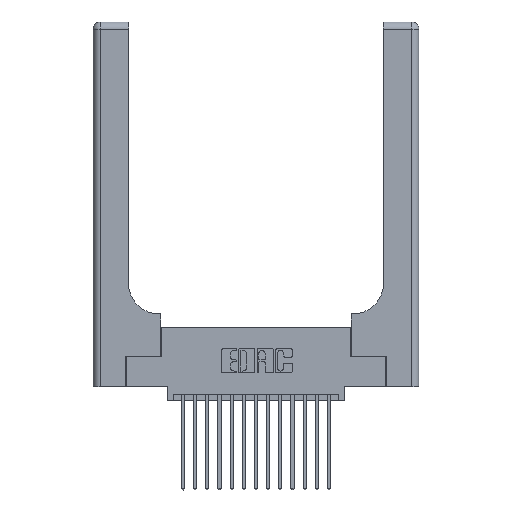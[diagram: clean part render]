
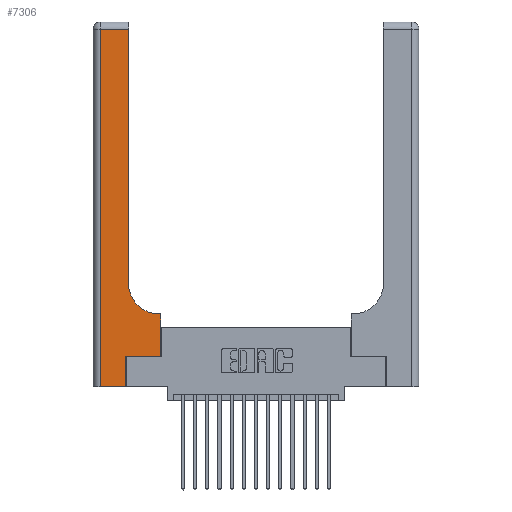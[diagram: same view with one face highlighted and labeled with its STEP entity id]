
A CAD part, top view. The second image highlights one B-rep face of the part: STEP entity #7306.
In plain terms, the highlighted planar face has unit normal (0, 0, 1).
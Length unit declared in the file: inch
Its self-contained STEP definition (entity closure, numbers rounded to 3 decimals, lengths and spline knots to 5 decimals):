
#80 = ORIENTED_EDGE ( 'NONE', *, *, #18007, .T. ) ;
#133 = CARTESIAN_POINT ( 'NONE',  ( 0.2915, 0.85, 0.37 ) ) ;
#310 = CARTESIAN_POINT ( 'NONE',  ( 0.5415, 0.6, 0.37 ) ) ;
#951 = VECTOR ( 'NONE', #5493, 39.37008 ) ;
#1789 = CARTESIAN_POINT ( 'NONE',  ( 0.269, 0., 0.37 ) ) ;
#2284 = LINE ( 'NONE', #10333, #10471 ) ;
#2875 = VECTOR ( 'NONE', #17183, 39.37008 ) ;
#3182 = VERTEX_POINT ( 'NONE', #1789 ) ;
#3317 = EDGE_CURVE ( 'NONE', #3914, #3883, #15483, .T. ) ;
#3883 = VERTEX_POINT ( 'NONE', #9594 ) ;
#3914 = VERTEX_POINT ( 'NONE', #18693 ) ;
#3948 = CARTESIAN_POINT ( 'NONE',  ( 0.5585, 0.25, 0.37 ) ) ;
#4792 = AXIS2_PLACEMENT_3D ( 'NONE', #16618, #9261, #6582 ) ;
#5071 = CARTESIAN_POINT ( 'NONE',  ( 0.2915, 2.94, 0.37 ) ) ;
#5115 = VERTEX_POINT ( 'NONE', #3948 ) ;
#5223 = FACE_OUTER_BOUND ( 'NONE', #6684, .T. ) ;
#5493 = DIRECTION ( 'NONE',  ( 0., 1., 0. ) ) ;
#5684 = ORIENTED_EDGE ( 'NONE', *, *, #13061, .T. ) ;
#6031 = DIRECTION ( 'NONE',  ( 0., 1., 0. ) ) ;
#6466 = CARTESIAN_POINT ( 'NONE',  ( 0.5585, 0.6, 0.37 ) ) ;
#6493 = CARTESIAN_POINT ( 'NONE',  ( 0., 0., 0.37 ) ) ;
#6582 = DIRECTION ( 'NONE',  ( 1., 0., 0. ) ) ;
#6594 = CARTESIAN_POINT ( 'NONE',  ( 0.269, 0.25, 0.37 ) ) ;
#6619 = CARTESIAN_POINT ( 'NONE',  ( 0., 3., 0.37 ) ) ;
#6684 = EDGE_LOOP ( 'NONE', ( #7973, #14461, #9759, #18737, #5684, #13299, #80, #12429, #9542 ) ) ;
#6760 = DIRECTION ( 'NONE',  ( 1., 0., 0. ) ) ;
#7249 = DIRECTION ( 'NONE',  ( -1., 0., 0. ) ) ;
#7306 = ADVANCED_FACE ( 'NONE', ( #5223 ), #15540, .F. ) ;
#7374 = EDGE_CURVE ( 'NONE', #9875, #18195, #12712, .T. ) ;
#7973 = ORIENTED_EDGE ( 'NONE', *, *, #11420, .T. ) ;
#8090 = DIRECTION ( 'NONE',  ( 1., 0., 0. ) ) ;
#8292 = CARTESIAN_POINT ( 'NONE',  ( 0.06, 3., 0.37 ) ) ;
#8516 = AXIS2_PLACEMENT_3D ( 'NONE', #6619, #12692, #11057 ) ;
#8570 = DIRECTION ( 'NONE',  ( -1., 0., 0. ) ) ;
#9261 = DIRECTION ( 'NONE',  ( 0., 0., -1. ) ) ;
#9511 = VECTOR ( 'NONE', #8570, 39.37008 ) ;
#9542 = ORIENTED_EDGE ( 'NONE', *, *, #7374, .T. ) ;
#9594 = CARTESIAN_POINT ( 'NONE',  ( 0.06, 0., 0.37 ) ) ;
#9759 = ORIENTED_EDGE ( 'NONE', *, *, #3317, .T. ) ;
#9875 = VERTEX_POINT ( 'NONE', #310 ) ;
#10333 = CARTESIAN_POINT ( 'NONE',  ( 0., 2.94, 0.37 ) ) ;
#10471 = VECTOR ( 'NONE', #7249, 39.37008 ) ;
#10490 = VECTOR ( 'NONE', #6760, 39.37008 ) ;
#10528 = VERTEX_POINT ( 'NONE', #6466 ) ;
#10738 = VERTEX_POINT ( 'NONE', #14190 ) ;
#10763 = VECTOR ( 'NONE', #17199, 39.37008 ) ;
#11023 = CARTESIAN_POINT ( 'NONE',  ( 0.5585, 0.25, 0.37 ) ) ;
#11057 = DIRECTION ( 'NONE',  ( -1., 0., 0. ) ) ;
#11420 = EDGE_CURVE ( 'NONE', #18195, #12894, #17581, .T. ) ;
#11782 = CARTESIAN_POINT ( 'NONE',  ( 0.2915, 0.6, 0.37 ) ) ;
#12429 = ORIENTED_EDGE ( 'NONE', *, *, #14574, .T. ) ;
#12692 = DIRECTION ( 'NONE',  ( 0., 0., -1. ) ) ;
#12712 = CIRCLE ( 'NONE', #4792, 0.25 ) ;
#12780 = LINE ( 'NONE', #11782, #9511 ) ;
#12894 = VERTEX_POINT ( 'NONE', #5071 ) ;
#13061 = EDGE_CURVE ( 'NONE', #3182, #10738, #13520, .T. ) ;
#13126 = CARTESIAN_POINT ( 'NONE',  ( 0.2915, 3., 0.37 ) ) ;
#13263 = EDGE_CURVE ( 'NONE', #3883, #3182, #16127, .T. ) ;
#13299 = ORIENTED_EDGE ( 'NONE', *, *, #15379, .T. ) ;
#13520 = LINE ( 'NONE', #16599, #18934 ) ;
#13576 = EDGE_CURVE ( 'NONE', #12894, #3914, #2284, .T. ) ;
#13652 = VECTOR ( 'NONE', #8090, 39.37008 ) ;
#13886 = LINE ( 'NONE', #6594, #13652 ) ;
#14190 = CARTESIAN_POINT ( 'NONE',  ( 0.269, 0.25, 0.37 ) ) ;
#14461 = ORIENTED_EDGE ( 'NONE', *, *, #13576, .T. ) ;
#14574 = EDGE_CURVE ( 'NONE', #10528, #9875, #12780, .T. ) ;
#15379 = EDGE_CURVE ( 'NONE', #10738, #5115, #13886, .T. ) ;
#15483 = LINE ( 'NONE', #8292, #10763 ) ;
#15540 = PLANE ( 'NONE',  #8516 ) ;
#16127 = LINE ( 'NONE', #6493, #10490 ) ;
#16599 = CARTESIAN_POINT ( 'NONE',  ( 0.269, 0., 0.37 ) ) ;
#16618 = CARTESIAN_POINT ( 'NONE',  ( 0.5415, 0.85, 0.37 ) ) ;
#17183 = DIRECTION ( 'NONE',  ( 0., 1., 0. ) ) ;
#17199 = DIRECTION ( 'NONE',  ( 0., -1., 0. ) ) ;
#17438 = LINE ( 'NONE', #11023, #2875 ) ;
#17581 = LINE ( 'NONE', #13126, #951 ) ;
#18007 = EDGE_CURVE ( 'NONE', #5115, #10528, #17438, .T. ) ;
#18195 = VERTEX_POINT ( 'NONE', #133 ) ;
#18693 = CARTESIAN_POINT ( 'NONE',  ( 0.06, 2.94, 0.37 ) ) ;
#18737 = ORIENTED_EDGE ( 'NONE', *, *, #13263, .T. ) ;
#18934 = VECTOR ( 'NONE', #6031, 39.37008 ) ;
